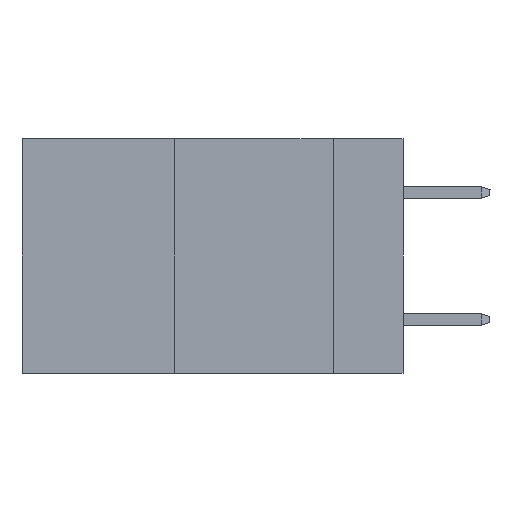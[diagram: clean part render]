
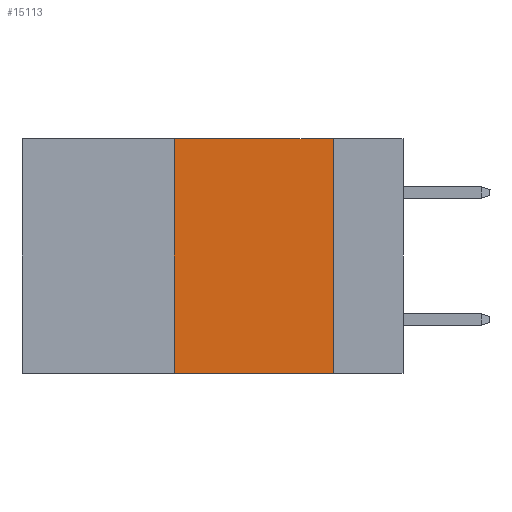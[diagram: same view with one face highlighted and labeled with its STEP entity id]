
A CAD part, left-side view. The second image highlights one B-rep face of the part: STEP entity #15113.
In plain terms, the highlighted planar face has unit normal (-1, 0, 0).
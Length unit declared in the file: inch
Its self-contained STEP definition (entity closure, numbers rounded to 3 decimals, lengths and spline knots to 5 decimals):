
#332 = LINE ( 'NONE', #6529, #4622 ) ;
#1535 = CARTESIAN_POINT ( 'NONE',  ( 0., 0.6, 0. ) ) ;
#1784 = CARTESIAN_POINT ( 'NONE',  ( 0., 0.6, -0.37 ) ) ;
#2132 = ORIENTED_EDGE ( 'NONE', *, *, #14350, .T. ) ;
#3216 = VERTEX_POINT ( 'NONE', #17023 ) ;
#3272 = DIRECTION ( 'NONE',  ( 0., 0., -1. ) ) ;
#3634 = CARTESIAN_POINT ( 'NONE',  ( 0., 0.11, 0. ) ) ;
#4622 = VECTOR ( 'NONE', #12720, 39.37008 ) ;
#5298 = EDGE_CURVE ( 'NONE', #15412, #19559, #332, .T. ) ;
#5387 = CARTESIAN_POINT ( 'NONE',  ( 0., 0.36, -0.37 ) ) ;
#6355 = CARTESIAN_POINT ( 'NONE',  ( 0., 0.11, -0.37 ) ) ;
#6380 = EDGE_CURVE ( 'NONE', #3216, #14294, #17544, .T. ) ;
#6529 = CARTESIAN_POINT ( 'NONE',  ( 0., 0.36, 0. ) ) ;
#6686 = VECTOR ( 'NONE', #7184, 39.37008 ) ;
#6725 = AXIS2_PLACEMENT_3D ( 'NONE', #1535, #15360, #3272 ) ;
#7184 = DIRECTION ( 'NONE',  ( 0., -1., 0. ) ) ;
#9277 = ORIENTED_EDGE ( 'NONE', *, *, #17361, .F. ) ;
#9423 = LINE ( 'NONE', #1784, #19163 ) ;
#10579 = FACE_OUTER_BOUND ( 'NONE', #14574, .T. ) ;
#12720 = DIRECTION ( 'NONE',  ( 0., 0., 1. ) ) ;
#14294 = VERTEX_POINT ( 'NONE', #6355 ) ;
#14350 = EDGE_CURVE ( 'NONE', #15412, #14294, #9423, .T. ) ;
#14574 = EDGE_LOOP ( 'NONE', ( #18110, #9277, #15867, #2132 ) ) ;
#14674 = CARTESIAN_POINT ( 'NONE',  ( 0., 0.36, 0. ) ) ;
#14806 = CARTESIAN_POINT ( 'NONE',  ( 0., 0.6, 0. ) ) ;
#15113 = ADVANCED_FACE ( 'NONE', ( #10579 ), #17196, .F. ) ;
#15354 = VECTOR ( 'NONE', #16031, 39.37008 ) ;
#15360 = DIRECTION ( 'NONE',  ( 1., 0., 0. ) ) ;
#15412 = VERTEX_POINT ( 'NONE', #5387 ) ;
#15867 = ORIENTED_EDGE ( 'NONE', *, *, #5298, .F. ) ;
#16031 = DIRECTION ( 'NONE',  ( 0., 0., -1. ) ) ;
#17023 = CARTESIAN_POINT ( 'NONE',  ( 0., 0.11, 0. ) ) ;
#17196 = PLANE ( 'NONE',  #6725 ) ;
#17361 = EDGE_CURVE ( 'NONE', #19559, #3216, #19686, .T. ) ;
#17544 = LINE ( 'NONE', #3634, #15354 ) ;
#18110 = ORIENTED_EDGE ( 'NONE', *, *, #6380, .F. ) ;
#18555 = DIRECTION ( 'NONE',  ( 0., -1., 0. ) ) ;
#19163 = VECTOR ( 'NONE', #18555, 39.37008 ) ;
#19559 = VERTEX_POINT ( 'NONE', #14674 ) ;
#19686 = LINE ( 'NONE', #14806, #6686 ) ;
